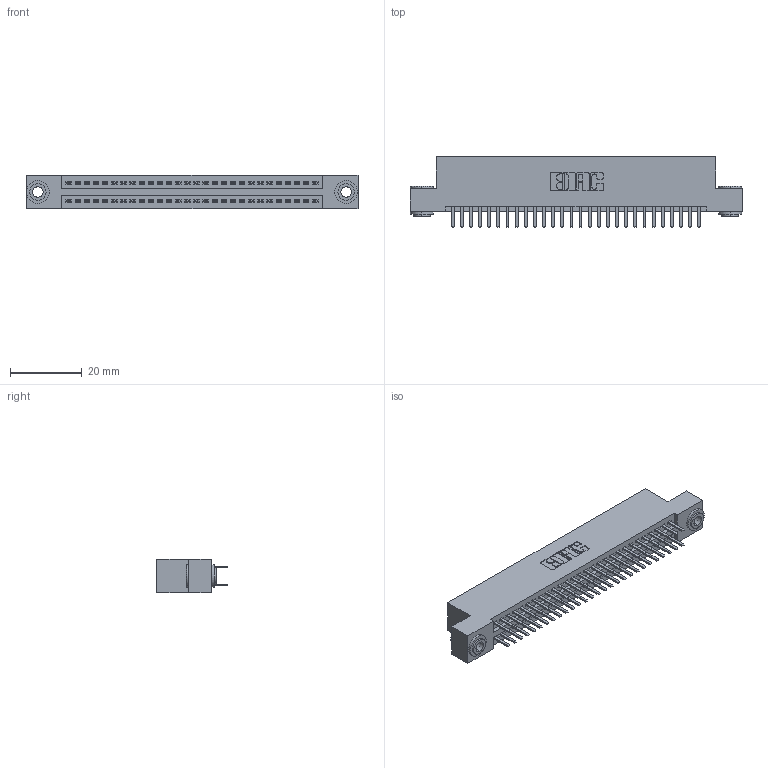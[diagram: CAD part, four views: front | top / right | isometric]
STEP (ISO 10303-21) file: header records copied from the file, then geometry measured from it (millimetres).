
FILE_DESCRIPTION (( 'STEP AP203' ), '1' );
FILE_NAME ('345-056-520-203.STEP', '2019-10-29T20:45:03', ( '' ), ( '' ), 'SwSTEP 2.0', 'SolidWorks 2016', '' );
FILE_SCHEMA (( 'CONFIG_CONTROL_DESIGN' ));
Length unit declared in the file: inch
Products named in the file (4): 345-056-520-203; 345 Part_Flush Mounting Lugs - 0.156 Dia-TH; 345-292-001_345-293-120; 345-250-002_345-250-002-102
Assembly tree (59 placements, depth 2):
  345-056-520-203
    345 Part_Flush Mounting Lugs - 0.156 Dia-TH
    345-292-001_345-293-120  x56
    345-250-002_345-250-002-102  x2
Bounding box: 92.33 x 19.68 x 9.4 mm (x, y, z)
Volume: 8833.8 mm3; surface area: 12939.2 mm2
Topology: 59 solids, 59 shells, 3188 faces, 9209 edges, 5986 vertices
Faces by surface type: plane 2050, cylinder 1130, cone 8
Entity records: 24618 total; most frequent: CARTESIAN_POINT 4127, ORIENTED_EDGE 4042, DIRECTION 3675, EDGE_CURVE 2021, VECTOR 1749, LINE 1749, VERTEX_POINT 1342, AXIS2_PLACEMENT_3D 963
